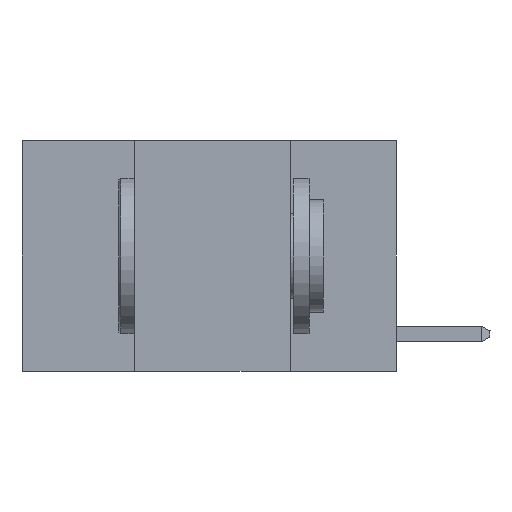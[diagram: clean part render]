
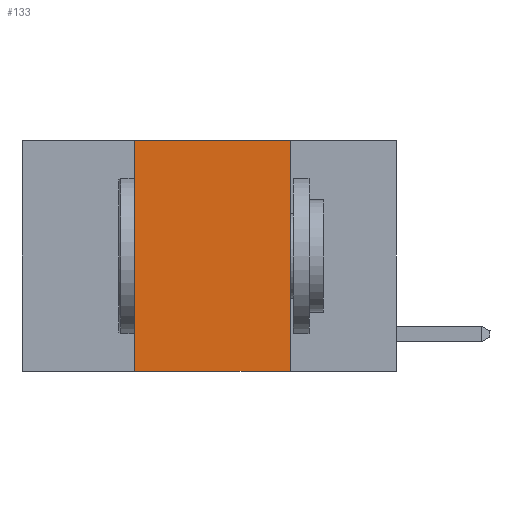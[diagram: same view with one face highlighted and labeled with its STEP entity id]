
A CAD part, left-side view. The second image highlights one B-rep face of the part: STEP entity #133.
In plain terms, the highlighted planar face has unit normal (-1, 0, 0).
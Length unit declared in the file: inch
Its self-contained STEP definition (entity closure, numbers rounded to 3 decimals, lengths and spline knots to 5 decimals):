
#133 = ADVANCED_FACE ( 'NONE', ( #8601 ), #8292, .F. ) ;
#675 = VECTOR ( 'NONE', #17344, 39.37008 ) ;
#1423 = CARTESIAN_POINT ( 'NONE',  ( 0., 0.17, 0. ) ) ;
#1893 = ORIENTED_EDGE ( 'NONE', *, *, #5246, .F. ) ;
#2087 = ORIENTED_EDGE ( 'NONE', *, *, #7188, .T. ) ;
#3830 = CARTESIAN_POINT ( 'NONE',  ( 0., 0.42, -0.37 ) ) ;
#4278 = LINE ( 'NONE', #4604, #6763 ) ;
#4400 = ORIENTED_EDGE ( 'NONE', *, *, #13703, .F. ) ;
#4604 = CARTESIAN_POINT ( 'NONE',  ( 0., 0.6, 0. ) ) ;
#5246 = EDGE_CURVE ( 'NONE', #16914, #9437, #4278, .T. ) ;
#5481 = EDGE_LOOP ( 'NONE', ( #19419, #1893, #4400, #2087 ) ) ;
#6196 = EDGE_CURVE ( 'NONE', #9437, #15541, #20850, .T. ) ;
#6763 = VECTOR ( 'NONE', #11069, 39.37008 ) ;
#7188 = EDGE_CURVE ( 'NONE', #11740, #15541, #19423, .T. ) ;
#7954 = DIRECTION ( 'NONE',  ( 0., -1., 0. ) ) ;
#8292 = PLANE ( 'NONE',  #20079 ) ;
#8601 = FACE_OUTER_BOUND ( 'NONE', #5481, .T. ) ;
#9437 = VERTEX_POINT ( 'NONE', #15984 ) ;
#10981 = VECTOR ( 'NONE', #20898, 39.37008 ) ;
#11069 = DIRECTION ( 'NONE',  ( 0., -1., 0. ) ) ;
#11740 = VERTEX_POINT ( 'NONE', #3830 ) ;
#12400 = CARTESIAN_POINT ( 'NONE',  ( 0., 0.17, -0.37 ) ) ;
#13044 = CARTESIAN_POINT ( 'NONE',  ( 0., 0.6, -0.37 ) ) ;
#13703 = EDGE_CURVE ( 'NONE', #11740, #16914, #17503, .T. ) ;
#13803 = CARTESIAN_POINT ( 'NONE',  ( 0., 0.6, 0. ) ) ;
#15541 = VERTEX_POINT ( 'NONE', #12400 ) ;
#15982 = VECTOR ( 'NONE', #7954, 39.37008 ) ;
#15984 = CARTESIAN_POINT ( 'NONE',  ( 0., 0.17, 0. ) ) ;
#16504 = CARTESIAN_POINT ( 'NONE',  ( 0., 0.42, 0. ) ) ;
#16914 = VERTEX_POINT ( 'NONE', #18704 ) ;
#17304 = DIRECTION ( 'NONE',  ( 0., 0., -1. ) ) ;
#17344 = DIRECTION ( 'NONE',  ( 0., 0., -1. ) ) ;
#17503 = LINE ( 'NONE', #16504, #10981 ) ;
#18704 = CARTESIAN_POINT ( 'NONE',  ( 0., 0.42, 0. ) ) ;
#19419 = ORIENTED_EDGE ( 'NONE', *, *, #6196, .F. ) ;
#19423 = LINE ( 'NONE', #13044, #15982 ) ;
#20079 = AXIS2_PLACEMENT_3D ( 'NONE', #13803, #20080, #17304 ) ;
#20080 = DIRECTION ( 'NONE',  ( 1., 0., 0. ) ) ;
#20850 = LINE ( 'NONE', #1423, #675 ) ;
#20898 = DIRECTION ( 'NONE',  ( 0., 0., 1. ) ) ;
